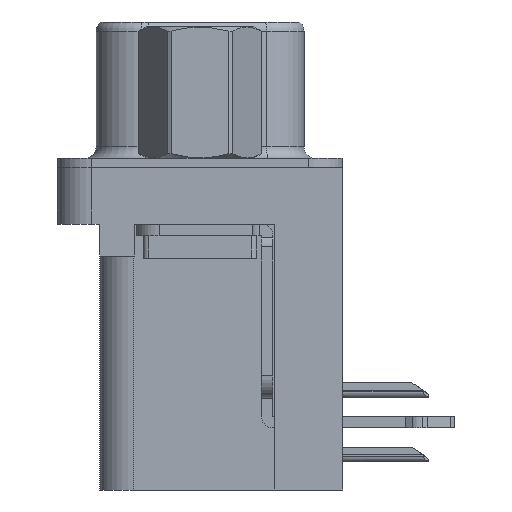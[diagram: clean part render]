
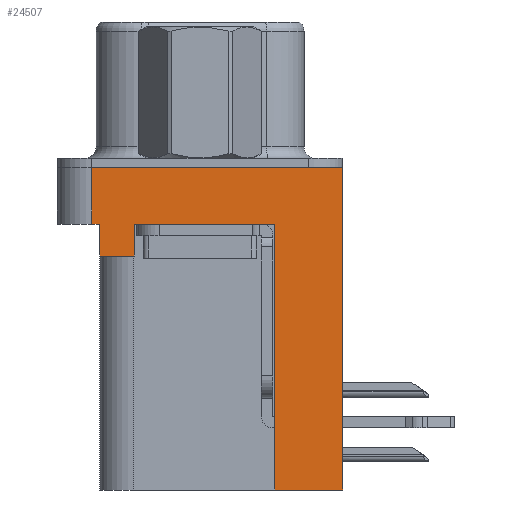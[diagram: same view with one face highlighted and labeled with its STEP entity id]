
A CAD part, left-side view. The second image highlights one B-rep face of the part: STEP entity #24507.
In plain terms, the highlighted planar face has unit normal (-1, 0, 0).
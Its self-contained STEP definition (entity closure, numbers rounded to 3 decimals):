
#1147 = ORIENTED_EDGE ( 'NONE', *, *, #20226, .F. ) ;
#1542 = VECTOR ( 'NONE', #11334, 1000. ) ;
#1635 = VECTOR ( 'NONE', #27057, 1000. ) ;
#2436 = CARTESIAN_POINT ( 'NONE',  ( -3., 2.895, -2.5 ) ) ;
#2638 = FACE_OUTER_BOUND ( 'NONE', #4105, .T. ) ;
#2755 = CARTESIAN_POINT ( 'NONE',  ( -3., -6.275, -2.5 ) ) ;
#2819 = EDGE_CURVE ( 'NONE', #24266, #5523, #27443, .T. ) ;
#2908 = DIRECTION ( 'NONE',  ( -1., 0., 0. ) ) ;
#3361 = VECTOR ( 'NONE', #14477, 1000. ) ;
#3651 = DIRECTION ( 'NONE',  ( 0., 0., 1. ) ) ;
#4105 = EDGE_LOOP ( 'NONE', ( #7243, #13193, #20661, #10940, #5057, #13577, #24405, #17449, #1147, #15839 ) ) ;
#4398 = EDGE_CURVE ( 'NONE', #19686, #27284, #27948, .T. ) ;
#5057 = ORIENTED_EDGE ( 'NONE', *, *, #4398, .F. ) ;
#5317 = VECTOR ( 'NONE', #16635, 1000. ) ;
#5523 = VERTEX_POINT ( 'NONE', #11095 ) ;
#5911 = CARTESIAN_POINT ( 'NONE',  ( -3., 4.425, -3.9 ) ) ;
#6090 = LINE ( 'NONE', #27699, #3361 ) ;
#6537 = VECTOR ( 'NONE', #25964, 1000. ) ;
#6619 = CARTESIAN_POINT ( 'NONE',  ( -3., -6.275, -2.5 ) ) ;
#6986 = VERTEX_POINT ( 'NONE', #25245 ) ;
#7029 = DIRECTION ( 'NONE',  ( 0., 0., 1. ) ) ;
#7243 = ORIENTED_EDGE ( 'NONE', *, *, #24024, .F. ) ;
#7510 = VERTEX_POINT ( 'NONE', #26443 ) ;
#8133 = CARTESIAN_POINT ( 'NONE',  ( -3., -6.275, -2.5 ) ) ;
#8333 = DIRECTION ( 'NONE',  ( 0., 1., 0. ) ) ;
#9299 = EDGE_CURVE ( 'NONE', #19686, #11224, #26101, .T. ) ;
#9695 = VERTEX_POINT ( 'NONE', #27776 ) ;
#10802 = CARTESIAN_POINT ( 'NONE',  ( -3., -6.275, 0. ) ) ;
#10838 = EDGE_CURVE ( 'NONE', #11224, #9695, #11554, .T. ) ;
#10887 = LINE ( 'NONE', #19539, #23355 ) ;
#10888 = CARTESIAN_POINT ( 'NONE',  ( -3., 2.895, -3.9 ) ) ;
#10890 = CARTESIAN_POINT ( 'NONE',  ( -3., 4.425, -3.9 ) ) ;
#10940 = ORIENTED_EDGE ( 'NONE', *, *, #13639, .F. ) ;
#11095 = CARTESIAN_POINT ( 'NONE',  ( -3., -6.275, 0. ) ) ;
#11224 = VERTEX_POINT ( 'NONE', #2436 ) ;
#11334 = DIRECTION ( 'NONE',  ( 0., 0., 1. ) ) ;
#11346 = VECTOR ( 'NONE', #3651, 1000. ) ;
#11554 = LINE ( 'NONE', #2755, #1635 ) ;
#13035 = VECTOR ( 'NONE', #26825, 1000. ) ;
#13193 = ORIENTED_EDGE ( 'NONE', *, *, #20506, .F. ) ;
#13577 = ORIENTED_EDGE ( 'NONE', *, *, #9299, .T. ) ;
#13639 = EDGE_CURVE ( 'NONE', #27284, #21445, #23118, .T. ) ;
#13713 = PLANE ( 'NONE',  #17511 ) ;
#14477 = DIRECTION ( 'NONE',  ( 0., 1., 0. ) ) ;
#15069 = LINE ( 'NONE', #10802, #13035 ) ;
#15828 = CARTESIAN_POINT ( 'NONE',  ( -3., 4.425, -3.9 ) ) ;
#15839 = ORIENTED_EDGE ( 'NONE', *, *, #2819, .T. ) ;
#16635 = DIRECTION ( 'NONE',  ( 0., 0., 1. ) ) ;
#17449 = ORIENTED_EDGE ( 'NONE', *, *, #20832, .F. ) ;
#17511 = AXIS2_PLACEMENT_3D ( 'NONE', #6619, #2908, #7029 ) ;
#18528 = EDGE_CURVE ( 'NONE', #18973, #21445, #27600, .T. ) ;
#18973 = VERTEX_POINT ( 'NONE', #27155 ) ;
#19539 = CARTESIAN_POINT ( 'NONE',  ( -3., -3.295, -14.2 ) ) ;
#19686 = VERTEX_POINT ( 'NONE', #26798 ) ;
#20226 = EDGE_CURVE ( 'NONE', #24266, #7510, #6090, .T. ) ;
#20506 = EDGE_CURVE ( 'NONE', #18973, #6986, #24551, .T. ) ;
#20640 = DIRECTION ( 'NONE',  ( 0., -1., 0. ) ) ;
#20661 = ORIENTED_EDGE ( 'NONE', *, *, #18528, .T. ) ;
#20832 = EDGE_CURVE ( 'NONE', #7510, #9695, #10887, .T. ) ;
#20867 = VECTOR ( 'NONE', #8333, 1000. ) ;
#21019 = CARTESIAN_POINT ( 'NONE',  ( -3., 4.425, -2.5 ) ) ;
#21445 = VERTEX_POINT ( 'NONE', #21019 ) ;
#23118 = LINE ( 'NONE', #5911, #11346 ) ;
#23355 = VECTOR ( 'NONE', #27668, 1000. ) ;
#24024 = EDGE_CURVE ( 'NONE', #6986, #5523, #15069, .T. ) ;
#24266 = VERTEX_POINT ( 'NONE', #27109 ) ;
#24280 = CARTESIAN_POINT ( 'NONE',  ( -3., 4.775, -2.5 ) ) ;
#24405 = ORIENTED_EDGE ( 'NONE', *, *, #10838, .T. ) ;
#24507 = ADVANCED_FACE ( 'NONE', ( #2638 ), #13713, .T. ) ;
#24551 = LINE ( 'NONE', #24280, #1542 ) ;
#25245 = CARTESIAN_POINT ( 'NONE',  ( -3., 4.775, 0. ) ) ;
#25460 = CARTESIAN_POINT ( 'NONE',  ( -3., -6.275, -2.5 ) ) ;
#25964 = DIRECTION ( 'NONE',  ( 0., 0., 1. ) ) ;
#26101 = LINE ( 'NONE', #10888, #6537 ) ;
#26443 = CARTESIAN_POINT ( 'NONE',  ( -3., -3.295, -14.2 ) ) ;
#26798 = CARTESIAN_POINT ( 'NONE',  ( -3., 2.895, -3.9 ) ) ;
#26825 = DIRECTION ( 'NONE',  ( 0., -1., 0. ) ) ;
#27057 = DIRECTION ( 'NONE',  ( 0., -1., 0. ) ) ;
#27109 = CARTESIAN_POINT ( 'NONE',  ( -3., -6.275, -14.2 ) ) ;
#27155 = CARTESIAN_POINT ( 'NONE',  ( -3., 4.775, -2.5 ) ) ;
#27284 = VERTEX_POINT ( 'NONE', #15828 ) ;
#27332 = VECTOR ( 'NONE', #20640, 1000. ) ;
#27443 = LINE ( 'NONE', #25460, #5317 ) ;
#27600 = LINE ( 'NONE', #8133, #27332 ) ;
#27668 = DIRECTION ( 'NONE',  ( 0., 0., 1. ) ) ;
#27699 = CARTESIAN_POINT ( 'NONE',  ( -3., -3.295, -14.2 ) ) ;
#27776 = CARTESIAN_POINT ( 'NONE',  ( -3., -3.295, -2.5 ) ) ;
#27948 = LINE ( 'NONE', #10890, #20867 ) ;
